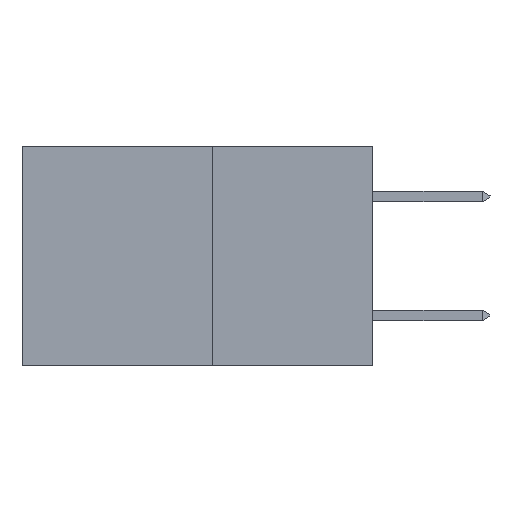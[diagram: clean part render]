
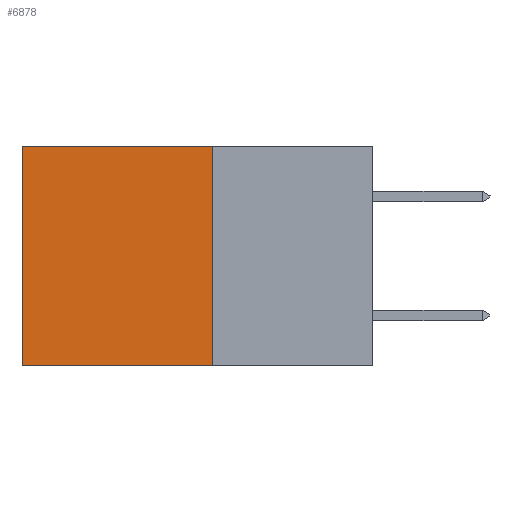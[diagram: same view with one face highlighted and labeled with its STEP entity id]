
A CAD part, left-side view. The second image highlights one B-rep face of the part: STEP entity #6878.
In plain terms, the highlighted planar face has unit normal (-1, 0, 0).
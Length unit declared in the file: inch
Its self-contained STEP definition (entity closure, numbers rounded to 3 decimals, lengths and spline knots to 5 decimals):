
#454 = CARTESIAN_POINT ( 'NONE',  ( 0.277, 0.59, -0.37 ) ) ;
#474 = DIRECTION ( 'NONE',  ( 1., 0., 0. ) ) ;
#794 = EDGE_CURVE ( 'NONE', #7943, #4463, #6280, .T. ) ;
#1934 = VECTOR ( 'NONE', #6368, 39.37008 ) ;
#2180 = ORIENTED_EDGE ( 'NONE', *, *, #5886, .T. ) ;
#3094 = LINE ( 'NONE', #6381, #6620 ) ;
#3403 = AXIS2_PLACEMENT_3D ( 'NONE', #5473, #474, #5504 ) ;
#3920 = ORIENTED_EDGE ( 'NONE', *, *, #5614, .F. ) ;
#4463 = VERTEX_POINT ( 'NONE', #8291 ) ;
#4768 = DIRECTION ( 'NONE',  ( 0., 1., 0. ) ) ;
#4793 = ORIENTED_EDGE ( 'NONE', *, *, #794, .T. ) ;
#4981 = CARTESIAN_POINT ( 'NONE',  ( 0.277, 0.27, 0. ) ) ;
#5042 = LINE ( 'NONE', #8655, #7610 ) ;
#5473 = CARTESIAN_POINT ( 'NONE',  ( 0.277, 0.27, -0.37 ) ) ;
#5504 = DIRECTION ( 'NONE',  ( 0., 0., -1. ) ) ;
#5614 = EDGE_CURVE ( 'NONE', #8856, #8118, #5042, .T. ) ;
#5886 = EDGE_CURVE ( 'NONE', #4463, #8118, #9035, .T. ) ;
#6280 = LINE ( 'NONE', #4981, #7864 ) ;
#6368 = DIRECTION ( 'NONE',  ( 0., 0., -1. ) ) ;
#6381 = CARTESIAN_POINT ( 'NONE',  ( 0.277, 0.27, -0.37 ) ) ;
#6489 = CARTESIAN_POINT ( 'NONE',  ( 0.277, 0.27, -0.37 ) ) ;
#6538 = ORIENTED_EDGE ( 'NONE', *, *, #8303, .F. ) ;
#6620 = VECTOR ( 'NONE', #7047, 39.37008 ) ;
#6762 = CARTESIAN_POINT ( 'NONE',  ( 0.277, 0.59, -0.37 ) ) ;
#6832 = EDGE_LOOP ( 'NONE', ( #2180, #3920, #6538, #4793 ) ) ;
#6878 = ADVANCED_FACE ( 'NONE', ( #7794 ), #8840, .F. ) ;
#7047 = DIRECTION ( 'NONE',  ( 0., 0., -1. ) ) ;
#7296 = CARTESIAN_POINT ( 'NONE',  ( 0.277, 0.27, 0. ) ) ;
#7610 = VECTOR ( 'NONE', #8409, 39.37008 ) ;
#7794 = FACE_OUTER_BOUND ( 'NONE', #6832, .T. ) ;
#7864 = VECTOR ( 'NONE', #4768, 39.37008 ) ;
#7943 = VERTEX_POINT ( 'NONE', #7296 ) ;
#8118 = VERTEX_POINT ( 'NONE', #454 ) ;
#8291 = CARTESIAN_POINT ( 'NONE',  ( 0.277, 0.59, 0. ) ) ;
#8303 = EDGE_CURVE ( 'NONE', #7943, #8856, #3094, .T. ) ;
#8409 = DIRECTION ( 'NONE',  ( 0., 1., 0. ) ) ;
#8655 = CARTESIAN_POINT ( 'NONE',  ( 0.277, 0.27, -0.37 ) ) ;
#8840 = PLANE ( 'NONE',  #3403 ) ;
#8856 = VERTEX_POINT ( 'NONE', #6489 ) ;
#9035 = LINE ( 'NONE', #6762, #1934 ) ;
